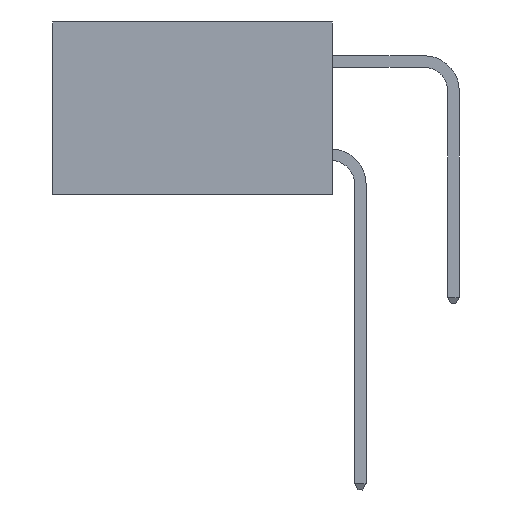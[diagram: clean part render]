
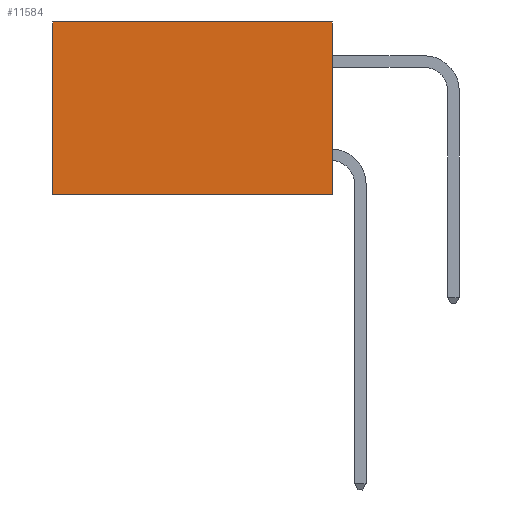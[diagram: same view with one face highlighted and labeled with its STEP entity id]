
A CAD part, left-side view. The second image highlights one B-rep face of the part: STEP entity #11584.
In plain terms, the highlighted planar face has unit normal (-1, 0, 0).
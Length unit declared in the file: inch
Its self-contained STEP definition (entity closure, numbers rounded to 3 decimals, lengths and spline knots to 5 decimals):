
#1066 = EDGE_LOOP ( 'NONE', ( #8371, #14075, #11922, #3797 ) ) ;
#1423 = CARTESIAN_POINT ( 'NONE',  ( 0.298, 0., -0.37 ) ) ;
#2015 = EDGE_CURVE ( 'NONE', #15690, #8882, #9034, .T. ) ;
#2714 = EDGE_CURVE ( 'NONE', #15446, #15067, #8405, .T. ) ;
#2890 = CARTESIAN_POINT ( 'NONE',  ( 0.298, 0.6, 0. ) ) ;
#3269 = EDGE_CURVE ( 'NONE', #8882, #15067, #7039, .T. ) ;
#3469 = EDGE_CURVE ( 'NONE', #15690, #15446, #14271, .T. ) ;
#3769 = VECTOR ( 'NONE', #11451, 39.37008 ) ;
#3797 = ORIENTED_EDGE ( 'NONE', *, *, #3469, .T. ) ;
#4034 = FACE_OUTER_BOUND ( 'NONE', #1066, .T. ) ;
#4228 = DIRECTION ( 'NONE',  ( 0., 1., 0. ) ) ;
#4325 = VECTOR ( 'NONE', #4228, 39.37008 ) ;
#5059 = DIRECTION ( 'NONE',  ( 1., 0., 0. ) ) ;
#7039 = LINE ( 'NONE', #1423, #3769 ) ;
#7351 = CARTESIAN_POINT ( 'NONE',  ( 0.298, 0., -0.37 ) ) ;
#8371 = ORIENTED_EDGE ( 'NONE', *, *, #2714, .T. ) ;
#8405 = LINE ( 'NONE', #9956, #14646 ) ;
#8694 = DIRECTION ( 'NONE',  ( 0., 0., -1. ) ) ;
#8882 = VERTEX_POINT ( 'NONE', #7351 ) ;
#9034 = LINE ( 'NONE', #14623, #9437 ) ;
#9437 = VECTOR ( 'NONE', #8694, 39.37008 ) ;
#9956 = CARTESIAN_POINT ( 'NONE',  ( 0.298, 0.6, 0. ) ) ;
#10048 = PLANE ( 'NONE',  #11528 ) ;
#10212 = DIRECTION ( 'NONE',  ( 0., 0., -1. ) ) ;
#11451 = DIRECTION ( 'NONE',  ( 0., 1., 0. ) ) ;
#11528 = AXIS2_PLACEMENT_3D ( 'NONE', #12579, #5059, #13801 ) ;
#11584 = ADVANCED_FACE ( 'NONE', ( #4034 ), #10048, .F. ) ;
#11706 = CARTESIAN_POINT ( 'NONE',  ( 0.298, 0., 0. ) ) ;
#11922 = ORIENTED_EDGE ( 'NONE', *, *, #2015, .F. ) ;
#12579 = CARTESIAN_POINT ( 'NONE',  ( 0.298, 0., 0. ) ) ;
#13801 = DIRECTION ( 'NONE',  ( 0., 0., -1. ) ) ;
#14075 = ORIENTED_EDGE ( 'NONE', *, *, #3269, .F. ) ;
#14271 = LINE ( 'NONE', #11706, #4325 ) ;
#14623 = CARTESIAN_POINT ( 'NONE',  ( 0.298, 0., 0. ) ) ;
#14646 = VECTOR ( 'NONE', #10212, 39.37008 ) ;
#15067 = VERTEX_POINT ( 'NONE', #15822 ) ;
#15446 = VERTEX_POINT ( 'NONE', #2890 ) ;
#15690 = VERTEX_POINT ( 'NONE', #15699 ) ;
#15699 = CARTESIAN_POINT ( 'NONE',  ( 0.298, 0., 0. ) ) ;
#15822 = CARTESIAN_POINT ( 'NONE',  ( 0.298, 0.6, -0.37 ) ) ;
